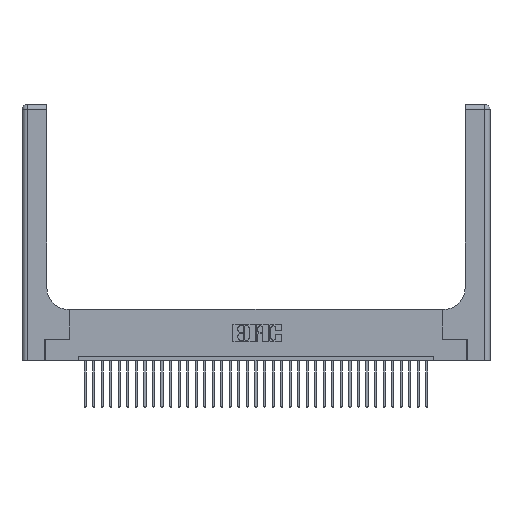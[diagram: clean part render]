
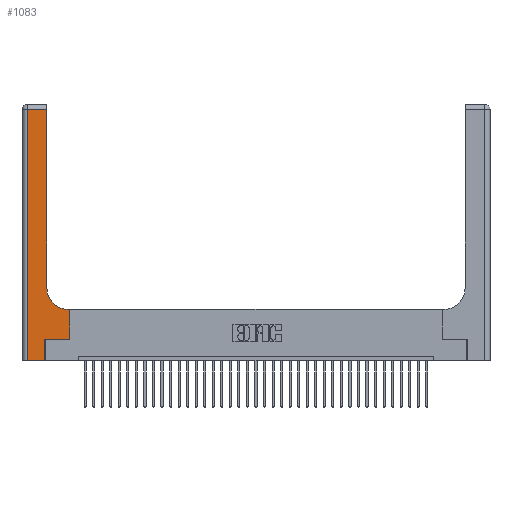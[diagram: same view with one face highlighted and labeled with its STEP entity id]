
A CAD part, top view. The second image highlights one B-rep face of the part: STEP entity #1083.
In plain terms, the highlighted planar face has unit normal (0, 0, 1).
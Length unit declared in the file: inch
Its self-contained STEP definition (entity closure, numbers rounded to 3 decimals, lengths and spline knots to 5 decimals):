
#815 = DIRECTION ( 'NONE',  ( -1., 0., 0. ) ) ;
#1083 = ADVANCED_FACE ( 'NONE', ( #29356 ), #5620, .F. ) ;
#1251 = CARTESIAN_POINT ( 'NONE',  ( 0.06, 3., 0.37 ) ) ;
#1817 = VECTOR ( 'NONE', #36182, 39.37008 ) ;
#2105 = LINE ( 'NONE', #1251, #13414 ) ;
#2471 = VECTOR ( 'NONE', #2654, 39.37008 ) ;
#2479 = CARTESIAN_POINT ( 'NONE',  ( 0.06, 2.94, 0.37 ) ) ;
#2645 = CARTESIAN_POINT ( 'NONE',  ( 0., 0., 0.37 ) ) ;
#2654 = DIRECTION ( 'NONE',  ( -1., 0., 0. ) ) ;
#2691 = ORIENTED_EDGE ( 'NONE', *, *, #11675, .T. ) ;
#2954 = CARTESIAN_POINT ( 'NONE',  ( 0.2915, 2.94, 0.37 ) ) ;
#3431 = VECTOR ( 'NONE', #25507, 39.37008 ) ;
#3862 = ORIENTED_EDGE ( 'NONE', *, *, #35432, .T. ) ;
#4420 = CARTESIAN_POINT ( 'NONE',  ( 0.2915, 0.85, 0.37 ) ) ;
#5571 = CARTESIAN_POINT ( 'NONE',  ( 0., 2.94, 0.37 ) ) ;
#5620 = PLANE ( 'NONE',  #7503 ) ;
#5813 = VECTOR ( 'NONE', #11411, 39.37008 ) ;
#6040 = EDGE_CURVE ( 'NONE', #7786, #28240, #20896, .T. ) ;
#6666 = LINE ( 'NONE', #28346, #5813 ) ;
#7005 = LINE ( 'NONE', #30373, #1817 ) ;
#7055 = CARTESIAN_POINT ( 'NONE',  ( 0.5585, 0.25, 0.37 ) ) ;
#7442 = DIRECTION ( 'NONE',  ( 0., -1., 0. ) ) ;
#7503 = AXIS2_PLACEMENT_3D ( 'NONE', #33586, #9133, #26026 ) ;
#7777 = ORIENTED_EDGE ( 'NONE', *, *, #28636, .T. ) ;
#7786 = VERTEX_POINT ( 'NONE', #26659 ) ;
#8076 = ORIENTED_EDGE ( 'NONE', *, *, #17884, .T. ) ;
#8401 = DIRECTION ( 'NONE',  ( 1., 0., 0. ) ) ;
#9133 = DIRECTION ( 'NONE',  ( 0., 0., -1. ) ) ;
#9399 = VERTEX_POINT ( 'NONE', #2954 ) ;
#9937 = CARTESIAN_POINT ( 'NONE',  ( 0.269, 0., 0.37 ) ) ;
#9969 = CARTESIAN_POINT ( 'NONE',  ( 0.269, 0., 0.37 ) ) ;
#10155 = EDGE_CURVE ( 'NONE', #14110, #9399, #6666, .T. ) ;
#10999 = VERTEX_POINT ( 'NONE', #20863 ) ;
#11411 = DIRECTION ( 'NONE',  ( 0., 1., 0. ) ) ;
#11675 = EDGE_CURVE ( 'NONE', #12585, #30999, #31086, .T. ) ;
#12585 = VERTEX_POINT ( 'NONE', #15126 ) ;
#13414 = VECTOR ( 'NONE', #7442, 39.37008 ) ;
#14016 = DIRECTION ( 'NONE',  ( 0., 0., -1. ) ) ;
#14110 = VERTEX_POINT ( 'NONE', #4420 ) ;
#14334 = ORIENTED_EDGE ( 'NONE', *, *, #35035, .T. ) ;
#15126 = CARTESIAN_POINT ( 'NONE',  ( 0.06, 0., 0.37 ) ) ;
#15579 = CIRCLE ( 'NONE', #28478, 0.25 ) ;
#15663 = DIRECTION ( 'NONE',  ( 0., 1., 0. ) ) ;
#15856 = VECTOR ( 'NONE', #815, 39.37008 ) ;
#16169 = VECTOR ( 'NONE', #19595, 39.37008 ) ;
#16914 = CARTESIAN_POINT ( 'NONE',  ( 0.269, 0.25, 0.37 ) ) ;
#17520 = ORIENTED_EDGE ( 'NONE', *, *, #33050, .T. ) ;
#17884 = EDGE_CURVE ( 'NONE', #28240, #23381, #7005, .T. ) ;
#18691 = EDGE_LOOP ( 'NONE', ( #22025, #17520, #14334, #2691, #35950, #34061, #8076, #7777, #3862 ) ) ;
#19595 = DIRECTION ( 'NONE',  ( 1., 0., 0. ) ) ;
#19626 = VECTOR ( 'NONE', #15663, 39.37008 ) ;
#20863 = CARTESIAN_POINT ( 'NONE',  ( 0.5415, 0.6, 0.37 ) ) ;
#20896 = LINE ( 'NONE', #16914, #3431 ) ;
#22025 = ORIENTED_EDGE ( 'NONE', *, *, #10155, .T. ) ;
#23313 = LINE ( 'NONE', #28943, #15856 ) ;
#23381 = VERTEX_POINT ( 'NONE', #28085 ) ;
#25162 = CARTESIAN_POINT ( 'NONE',  ( 0.5415, 0.85, 0.37 ) ) ;
#25507 = DIRECTION ( 'NONE',  ( 1., 0., 0. ) ) ;
#26026 = DIRECTION ( 'NONE',  ( -1., 0., 0. ) ) ;
#26659 = CARTESIAN_POINT ( 'NONE',  ( 0.269, 0.25, 0.37 ) ) ;
#27956 = VERTEX_POINT ( 'NONE', #2479 ) ;
#28085 = CARTESIAN_POINT ( 'NONE',  ( 0.5585, 0.6, 0.37 ) ) ;
#28240 = VERTEX_POINT ( 'NONE', #7055 ) ;
#28346 = CARTESIAN_POINT ( 'NONE',  ( 0.2915, 3., 0.37 ) ) ;
#28478 = AXIS2_PLACEMENT_3D ( 'NONE', #25162, #14016, #8401 ) ;
#28636 = EDGE_CURVE ( 'NONE', #23381, #10999, #23313, .T. ) ;
#28943 = CARTESIAN_POINT ( 'NONE',  ( 0.2915, 0.6, 0.37 ) ) ;
#29356 = FACE_OUTER_BOUND ( 'NONE', #18691, .T. ) ;
#29585 = LINE ( 'NONE', #5571, #2471 ) ;
#30373 = CARTESIAN_POINT ( 'NONE',  ( 0.5585, 0.25, 0.37 ) ) ;
#30999 = VERTEX_POINT ( 'NONE', #9969 ) ;
#31086 = LINE ( 'NONE', #2645, #16169 ) ;
#31566 = EDGE_CURVE ( 'NONE', #30999, #7786, #33184, .T. ) ;
#33050 = EDGE_CURVE ( 'NONE', #9399, #27956, #29585, .T. ) ;
#33184 = LINE ( 'NONE', #9937, #19626 ) ;
#33586 = CARTESIAN_POINT ( 'NONE',  ( 0., 3., 0.37 ) ) ;
#34061 = ORIENTED_EDGE ( 'NONE', *, *, #6040, .T. ) ;
#35035 = EDGE_CURVE ( 'NONE', #27956, #12585, #2105, .T. ) ;
#35432 = EDGE_CURVE ( 'NONE', #10999, #14110, #15579, .T. ) ;
#35950 = ORIENTED_EDGE ( 'NONE', *, *, #31566, .T. ) ;
#36182 = DIRECTION ( 'NONE',  ( 0., 1., 0. ) ) ;
